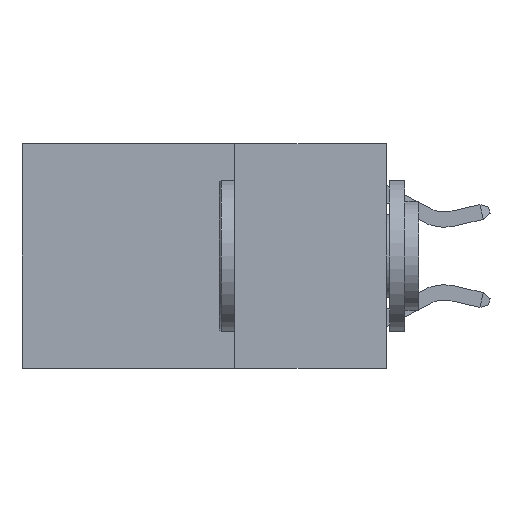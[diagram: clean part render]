
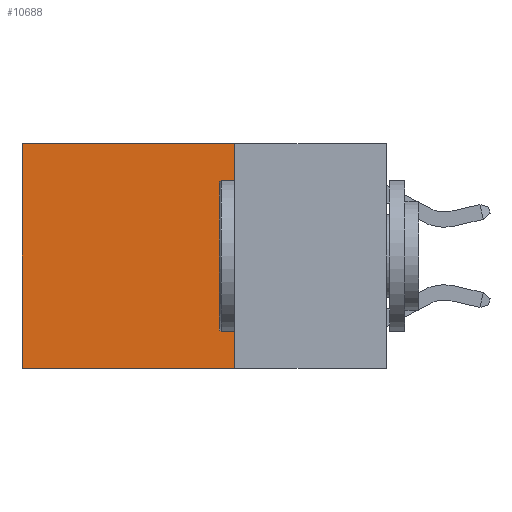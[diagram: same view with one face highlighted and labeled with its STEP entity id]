
A CAD part, left-side view. The second image highlights one B-rep face of the part: STEP entity #10688.
In plain terms, the highlighted planar face has unit normal (-1, 0, 0).
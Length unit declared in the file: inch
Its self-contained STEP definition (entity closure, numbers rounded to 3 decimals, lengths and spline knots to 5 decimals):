
#1391 = VERTEX_POINT ( 'NONE', #24866 ) ;
#1435 = ORIENTED_EDGE ( 'NONE', *, *, #21001, .F. ) ;
#1914 = VERTEX_POINT ( 'NONE', #18025 ) ;
#2013 = DIRECTION ( 'NONE',  ( 0., 0., -1. ) ) ;
#3066 = ORIENTED_EDGE ( 'NONE', *, *, #7948, .T. ) ;
#4148 = PLANE ( 'NONE',  #5388 ) ;
#4576 = CARTESIAN_POINT ( 'NONE',  ( 0.2625, 0.6, 0. ) ) ;
#5319 = VERTEX_POINT ( 'NONE', #10758 ) ;
#5388 = AXIS2_PLACEMENT_3D ( 'NONE', #19552, #7845, #2013 ) ;
#5472 = VECTOR ( 'NONE', #20742, 39.37008 ) ;
#6024 = LINE ( 'NONE', #9718, #10011 ) ;
#6579 = LINE ( 'NONE', #8732, #20796 ) ;
#6823 = DIRECTION ( 'NONE',  ( 0., 0., -1. ) ) ;
#6831 = ORIENTED_EDGE ( 'NONE', *, *, #23613, .T. ) ;
#7845 = DIRECTION ( 'NONE',  ( 1., 0., 0. ) ) ;
#7948 = EDGE_CURVE ( 'NONE', #20843, #5319, #6579, .T. ) ;
#8732 = CARTESIAN_POINT ( 'NONE',  ( 0.2625, 0.6, 0. ) ) ;
#9718 = CARTESIAN_POINT ( 'NONE',  ( 0.2625, 0.25, 0. ) ) ;
#10011 = VECTOR ( 'NONE', #13808, 39.37008 ) ;
#10688 = ADVANCED_FACE ( 'NONE', ( #21217 ), #4148, .F. ) ;
#10758 = CARTESIAN_POINT ( 'NONE',  ( 0.2625, 0.6, -0.37 ) ) ;
#12984 = CARTESIAN_POINT ( 'NONE',  ( 0.2625, 0.25, -0.37 ) ) ;
#13808 = DIRECTION ( 'NONE',  ( 0., 1., 0. ) ) ;
#14899 = VECTOR ( 'NONE', #6823, 39.37008 ) ;
#14984 = LINE ( 'NONE', #22721, #14899 ) ;
#15446 = EDGE_CURVE ( 'NONE', #1914, #1391, #14984, .T. ) ;
#16131 = DIRECTION ( 'NONE',  ( 0., 0., -1. ) ) ;
#17727 = EDGE_LOOP ( 'NONE', ( #3066, #1435, #19943, #6831 ) ) ;
#18025 = CARTESIAN_POINT ( 'NONE',  ( 0.2625, 0.25, 0. ) ) ;
#19552 = CARTESIAN_POINT ( 'NONE',  ( 0.2625, 0.25, 0. ) ) ;
#19943 = ORIENTED_EDGE ( 'NONE', *, *, #15446, .F. ) ;
#20742 = DIRECTION ( 'NONE',  ( 0., 1., 0. ) ) ;
#20796 = VECTOR ( 'NONE', #16131, 39.37008 ) ;
#20843 = VERTEX_POINT ( 'NONE', #4576 ) ;
#21001 = EDGE_CURVE ( 'NONE', #1391, #5319, #22635, .T. ) ;
#21217 = FACE_OUTER_BOUND ( 'NONE', #17727, .T. ) ;
#22635 = LINE ( 'NONE', #12984, #5472 ) ;
#22721 = CARTESIAN_POINT ( 'NONE',  ( 0.2625, 0.25, 0. ) ) ;
#23613 = EDGE_CURVE ( 'NONE', #1914, #20843, #6024, .T. ) ;
#24866 = CARTESIAN_POINT ( 'NONE',  ( 0.2625, 0.25, -0.37 ) ) ;
